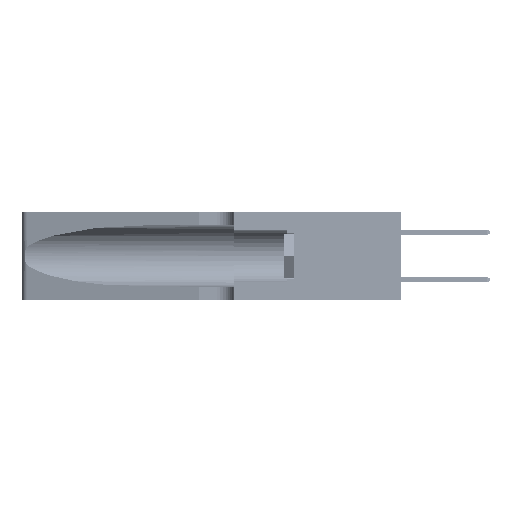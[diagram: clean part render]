
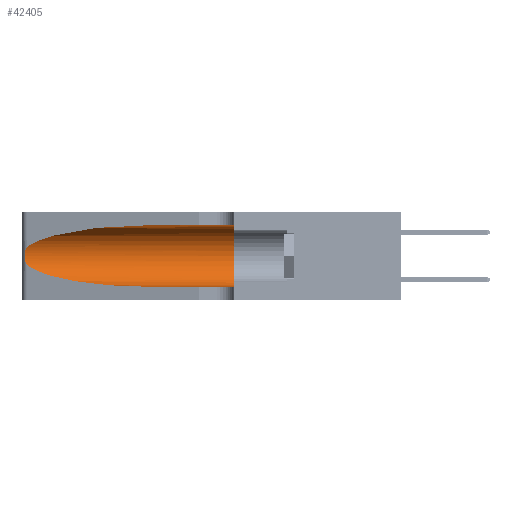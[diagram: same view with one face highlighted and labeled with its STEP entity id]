
A CAD part, left-side view. The second image highlights one B-rep face of the part: STEP entity #42405.
In plain terms, the highlighted cylindrical face has radius 3.308 mm (diameter 6.617 mm), a partial arc.
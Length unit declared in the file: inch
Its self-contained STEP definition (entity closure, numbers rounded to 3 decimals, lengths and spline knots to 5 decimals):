
#364 = CARTESIAN_POINT ( 'NONE',  ( 0.25854, 1.2359, 0.20912 ) ) ;
#402 = CARTESIAN_POINT ( 'NONE',  ( 0.1305, 0.72297, 0.31525 ) ) ;
#2689 = CARTESIAN_POINT ( 'NONE',  ( 0.1305, 0.35, 0.185 ) ) ;
#3571 =( BOUNDED_CURVE ( )  B_SPLINE_CURVE ( 3, ( #34988, #30796, #44398, #19357 ),
 .UNSPECIFIED., .F., .T. ) 
 B_SPLINE_CURVE_WITH_KNOTS ( ( 4, 4 ),
 ( 3.44316, 4.71239 ),
 .UNSPECIFIED. ) 
 CURVE ( )  GEOMETRIC_REPRESENTATION_ITEM ( )  RATIONAL_B_SPLINE_CURVE ( ( 1., 0.87, 0.87, 1. ) ) 
 REPRESENTATION_ITEM ( '' )  );
#4513 = CARTESIAN_POINT ( 'NONE',  ( 0.1305, 0.72297, 0.31525 ) ) ;
#4623 = CARTESIAN_POINT ( 'NONE',  ( 0.26075, 1.23896, 0.19203 ) ) ;
#5916 = LINE ( 'NONE', #13914, #26893 ) ;
#6899 = DIRECTION ( 'NONE',  ( 0., 0., 1. ) ) ;
#7608 = DIRECTION ( 'NONE',  ( 0., -1., 0. ) ) ;
#8722 = CARTESIAN_POINT ( 'NONE',  ( 0.25487, 1.22718, 0.22369 ) ) ;
#8829 = CARTESIAN_POINT ( 'NONE',  ( 0.26017, 1.23833, 0.17102 ) ) ;
#9271 = EDGE_CURVE ( 'NONE', #29376, #24836, #23295, .T. ) ;
#9596 = EDGE_CURVE ( 'NONE', #51658, #20496, #17357, .T. ) ;
#13033 = CARTESIAN_POINT ( 'NONE',  ( 0.25789, 1.23486, 0.15765 ) ) ;
#13332 = B_SPLINE_CURVE_WITH_KNOTS ( 'NONE', 3,
 ( #17070, #21314, #50472, #25532, #364, #29726, #4623, #33906, #8829, #38111, #13033, #42248, #17251, #46484 ),
 .UNSPECIFIED., .F., .F.,
 ( 4, 2, 2, 2, 2, 2, 4 ),
 ( 0., 0.00027, 0.00053, 0.00107, 0.0016, 0.00187, 0.00214 ),
 .UNSPECIFIED. ) ;
#13914 = CARTESIAN_POINT ( 'NONE',  ( 0.1305, 1.61858, 0.05475 ) ) ;
#14622 = CARTESIAN_POINT ( 'NONE',  ( 0.1305, 1.61858, 0.31525 ) ) ;
#14813 = CARTESIAN_POINT ( 'NONE',  ( 0.1305, 0.72297, 0.05475 ) ) ;
#16835 = ORIENTED_EDGE ( 'NONE', *, *, #9271, .F. ) ;
#17070 = CARTESIAN_POINT ( 'NONE',  ( 0.25487, 1.22718, 0.22369 ) ) ;
#17251 = CARTESIAN_POINT ( 'NONE',  ( 0.25555, 1.22993, 0.14849 ) ) ;
#17357 =( BOUNDED_CURVE ( )  B_SPLINE_CURVE ( 3, ( #4513, #25430, #21208, #8722 ),
 .UNSPECIFIED., .F., .F. ) 
 B_SPLINE_CURVE_WITH_KNOTS ( ( 4, 4 ),
 ( 1.5708, 2.84003 ),
 .UNSPECIFIED. ) 
 CURVE ( )  GEOMETRIC_REPRESENTATION_ITEM ( )  RATIONAL_B_SPLINE_CURVE ( ( 1., 0.87, 0.87, 1. ) ) 
 REPRESENTATION_ITEM ( '' )  );
#17997 = ORIENTED_EDGE ( 'NONE', *, *, #23660, .F. ) ;
#18247 = CARTESIAN_POINT ( 'NONE',  ( 0.25487, 1.22718, 0.14631 ) ) ;
#19062 = CYLINDRICAL_SURFACE ( 'NONE', #41008, 0.13025 ) ;
#19357 = CARTESIAN_POINT ( 'NONE',  ( 0.1305, 0.72297, 0.05475 ) ) ;
#19768 = VERTEX_POINT ( 'NONE', #14813 ) ;
#20058 = CARTESIAN_POINT ( 'NONE',  ( 0.1305, 1.61858, 0.185 ) ) ;
#20496 = VERTEX_POINT ( 'NONE', #34034 ) ;
#21208 = CARTESIAN_POINT ( 'NONE',  ( 0.2373, 1.15595, 0.28018 ) ) ;
#21314 = CARTESIAN_POINT ( 'NONE',  ( 0.25555, 1.22994, 0.2215 ) ) ;
#23295 = CIRCLE ( 'NONE', #52494, 0.13025 ) ;
#23660 = EDGE_CURVE ( 'NONE', #51658, #29376, #46666, .T. ) ;
#24836 = VERTEX_POINT ( 'NONE', #42668 ) ;
#25430 = CARTESIAN_POINT ( 'NONE',  ( 0.18966, 0.96281, 0.31525 ) ) ;
#25532 = CARTESIAN_POINT ( 'NONE',  ( 0.25787, 1.23484, 0.2124 ) ) ;
#26893 = VECTOR ( 'NONE', #34947, 39.37008 ) ;
#29376 = VERTEX_POINT ( 'NONE', #31008 ) ;
#29726 = CARTESIAN_POINT ( 'NONE',  ( 0.26018, 1.23835, 0.19895 ) ) ;
#30796 = CARTESIAN_POINT ( 'NONE',  ( 0.2373, 1.15595, 0.08982 ) ) ;
#31008 = CARTESIAN_POINT ( 'NONE',  ( 0.1305, 0.35, 0.31525 ) ) ;
#31998 = DIRECTION ( 'NONE',  ( 0., 1., 0. ) ) ;
#33906 = CARTESIAN_POINT ( 'NONE',  ( 0.26075, 1.23896, 0.178 ) ) ;
#34034 = CARTESIAN_POINT ( 'NONE',  ( 0.25487, 1.22718, 0.22369 ) ) ;
#34947 = DIRECTION ( 'NONE',  ( 0., -1., 0. ) ) ;
#34988 = CARTESIAN_POINT ( 'NONE',  ( 0.25487, 1.22718, 0.14631 ) ) ;
#35572 = VECTOR ( 'NONE', #52209, 39.37008 ) ;
#38002 = ORIENTED_EDGE ( 'NONE', *, *, #9596, .T. ) ;
#38111 = CARTESIAN_POINT ( 'NONE',  ( 0.25856, 1.23593, 0.16098 ) ) ;
#38916 = EDGE_CURVE ( 'NONE', #19768, #24836, #5916, .T. ) ;
#39601 = VERTEX_POINT ( 'NONE', #18247 ) ;
#40419 = ORIENTED_EDGE ( 'NONE', *, *, #38916, .T. ) ;
#41008 = AXIS2_PLACEMENT_3D ( 'NONE', #20058, #7608, #53415 ) ;
#42248 = CARTESIAN_POINT ( 'NONE',  ( 0.25639, 1.23186, 0.15144 ) ) ;
#42405 = ADVANCED_FACE ( 'NONE', ( #42614 ), #19062, .F. ) ;
#42614 = FACE_OUTER_BOUND ( 'NONE', #45257, .T. ) ;
#42668 = CARTESIAN_POINT ( 'NONE',  ( 0.1305, 0.35, 0.05475 ) ) ;
#44318 = ORIENTED_EDGE ( 'NONE', *, *, #50608, .T. ) ;
#44398 = CARTESIAN_POINT ( 'NONE',  ( 0.18966, 0.96281, 0.05475 ) ) ;
#45257 = EDGE_LOOP ( 'NONE', ( #38002, #44318, #52768, #40419, #16835, #17997 ) ) ;
#46484 = CARTESIAN_POINT ( 'NONE',  ( 0.25487, 1.22718, 0.14631 ) ) ;
#46666 = LINE ( 'NONE', #14622, #35572 ) ;
#50472 = CARTESIAN_POINT ( 'NONE',  ( 0.25639, 1.23184, 0.21858 ) ) ;
#50608 = EDGE_CURVE ( 'NONE', #20496, #39601, #13332, .T. ) ;
#50783 = EDGE_CURVE ( 'NONE', #39601, #19768, #3571, .T. ) ;
#51658 = VERTEX_POINT ( 'NONE', #402 ) ;
#52209 = DIRECTION ( 'NONE',  ( 0., -1., 0. ) ) ;
#52494 = AXIS2_PLACEMENT_3D ( 'NONE', #2689, #31998, #6899 ) ;
#52768 = ORIENTED_EDGE ( 'NONE', *, *, #50783, .T. ) ;
#53415 = DIRECTION ( 'NONE',  ( 0., 0., -1. ) ) ;
